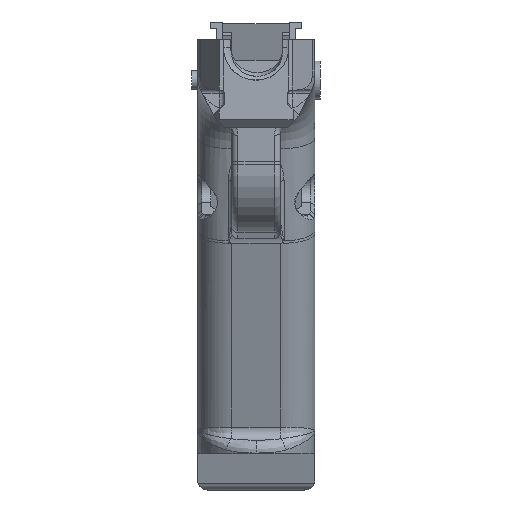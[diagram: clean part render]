
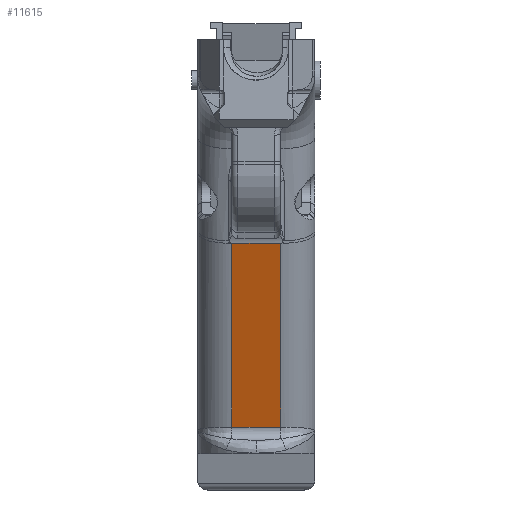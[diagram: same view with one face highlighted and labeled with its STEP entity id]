
A CAD part, front view. The second image highlights one B-rep face of the part: STEP entity #11615.
In plain terms, the highlighted planar face has unit normal (0, -0.947, -0.322).
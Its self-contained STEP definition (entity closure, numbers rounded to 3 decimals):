
#1335=FACE_OUTER_BOUND('',#1980,.T.);
#1980=EDGE_LOOP('',(#9789,#9790,#9791,#9792));
#2865=LINE('',#19617,#4048);
#3012=LINE('',#22087,#4195);
#3013=LINE('',#22095,#4196);
#3014=LINE('',#22096,#4197);
#4048=VECTOR('',#14401,10.);
#4195=VECTOR('',#14792,10.);
#4196=VECTOR('',#14795,10.);
#4197=VECTOR('',#14796,10.);
#5190=VERTEX_POINT('',#19610);
#5191=VERTEX_POINT('',#19616);
#5376=VERTEX_POINT('',#22079);
#5377=VERTEX_POINT('',#22086);
#6643=EDGE_CURVE('',#5190,#5191,#2865,.T.);
#6932=EDGE_CURVE('',#5376,#5377,#3012,.T.);
#6934=EDGE_CURVE('',#5377,#5190,#3013,.T.);
#6935=EDGE_CURVE('',#5191,#5376,#3014,.T.);
#9789=ORIENTED_EDGE('',*,*,#6643,.F.);
#9790=ORIENTED_EDGE('',*,*,#6934,.F.);
#9791=ORIENTED_EDGE('',*,*,#6932,.F.);
#9792=ORIENTED_EDGE('',*,*,#6935,.F.);
#11046=PLANE('',#12478);
#11615=ADVANCED_FACE('',(#1335),#11046,.T.);
#12478=AXIS2_PLACEMENT_3D('',#22094,#14793,#14794);
#14401=DIRECTION('',(-1.,0.,0.));
#14792=DIRECTION('',(1.,0.,0.));
#14793=DIRECTION('center_axis',(0.,-0.947,-0.322));
#14794=DIRECTION('ref_axis',(0.,0.322,-0.947));
#14795=DIRECTION('',(0.,0.322,-0.947));
#14796=DIRECTION('',(0.,-0.322,0.947));
#19610=CARTESIAN_POINT('',(-2.118,-62.644,-85.79));
#19616=CARTESIAN_POINT('',(-14.218,-62.644,-85.79));
#19617=CARTESIAN_POINT('',(-15.418,-62.644,-85.79));
#22079=CARTESIAN_POINT('',(-14.218,-78.109,-40.345));
#22086=CARTESIAN_POINT('',(-2.118,-78.109,-40.345));
#22087=CARTESIAN_POINT('',(0.,-78.109,-40.345));
#22094=CARTESIAN_POINT('Origin',(-22.668,-78.109,-40.345));
#22095=CARTESIAN_POINT('',(-2.118,-83.303,-25.083));
#22096=CARTESIAN_POINT('',(-14.218,-83.303,-25.083));
